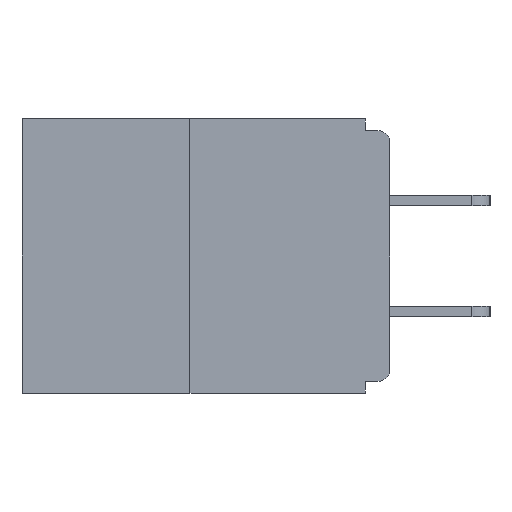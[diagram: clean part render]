
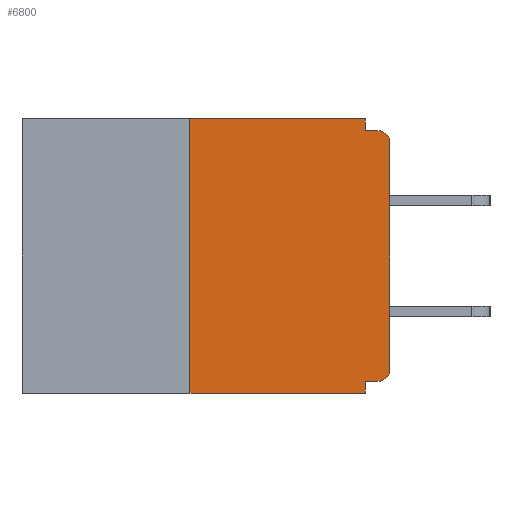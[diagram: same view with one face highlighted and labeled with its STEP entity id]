
A CAD part, left-side view. The second image highlights one B-rep face of the part: STEP entity #6800.
In plain terms, the highlighted planar face has unit normal (-1, 0, 0).
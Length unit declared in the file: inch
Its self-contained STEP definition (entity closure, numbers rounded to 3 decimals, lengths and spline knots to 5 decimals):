
#405 = DIRECTION ( 'NONE',  ( 0., -1., 0. ) ) ;
#660 = EDGE_CURVE ( 'NONE', #5271, #11070, #5580, .T. ) ;
#1061 = ORIENTED_EDGE ( 'NONE', *, *, #18727, .T. ) ;
#1547 = CARTESIAN_POINT ( 'NONE',  ( 0., 0.031, -0.015 ) ) ;
#1604 = DIRECTION ( 'NONE',  ( 0., 0., -1. ) ) ;
#2014 = AXIS2_PLACEMENT_3D ( 'NONE', #5248, #11078, #9657 ) ;
#2250 = VECTOR ( 'NONE', #5991, 39.37008 ) ;
#2292 = ORIENTED_EDGE ( 'NONE', *, *, #6930, .T. ) ;
#2561 = PLANE ( 'NONE',  #9073 ) ;
#3020 = CARTESIAN_POINT ( 'NONE',  ( 0., 0.015, -0.313 ) ) ;
#3096 = EDGE_CURVE ( 'NONE', #10043, #10060, #14631, .T. ) ;
#3568 = LINE ( 'NONE', #4851, #5735 ) ;
#3591 = ORIENTED_EDGE ( 'NONE', *, *, #660, .T. ) ;
#3662 = VECTOR ( 'NONE', #7138, 39.37008 ) ;
#3813 = EDGE_CURVE ( 'NONE', #8362, #7101, #16430, .T. ) ;
#4395 = EDGE_CURVE ( 'NONE', #10060, #13598, #16961, .T. ) ;
#4552 = CARTESIAN_POINT ( 'NONE',  ( 0., 0.46, 0. ) ) ;
#4698 = ORIENTED_EDGE ( 'NONE', *, *, #3096, .F. ) ;
#4843 = LINE ( 'NONE', #4552, #2250 ) ;
#4851 = CARTESIAN_POINT ( 'NONE',  ( 0., 0.031, 0. ) ) ;
#5020 = CARTESIAN_POINT ( 'NONE',  ( 0., 0.25, 0. ) ) ;
#5248 = CARTESIAN_POINT ( 'NONE',  ( 0., 0.015, -0.03 ) ) ;
#5271 = VERTEX_POINT ( 'NONE', #17336 ) ;
#5580 = LINE ( 'NONE', #8769, #11493 ) ;
#5625 = DIRECTION ( 'NONE',  ( 1., 0., 0. ) ) ;
#5735 = VECTOR ( 'NONE', #15248, 39.37008 ) ;
#5991 = DIRECTION ( 'NONE',  ( 0., -1., 0. ) ) ;
#6041 = ORIENTED_EDGE ( 'NONE', *, *, #9148, .T. ) ;
#6800 = ADVANCED_FACE ( 'NONE', ( #18742 ), #2561, .F. ) ;
#6930 = EDGE_CURVE ( 'NONE', #11070, #7101, #14533, .T. ) ;
#6936 = CIRCLE ( 'NONE', #8808, 0.015 ) ;
#6983 = CARTESIAN_POINT ( 'NONE',  ( 0., 0.031, -0.328 ) ) ;
#7101 = VERTEX_POINT ( 'NONE', #8712 ) ;
#7138 = DIRECTION ( 'NONE',  ( 0., -1., 0. ) ) ;
#7335 = CARTESIAN_POINT ( 'NONE',  ( 0., 0.46, -0.343 ) ) ;
#7573 = CARTESIAN_POINT ( 'NONE',  ( 0., 0., -0.328 ) ) ;
#7575 = ORIENTED_EDGE ( 'NONE', *, *, #3813, .F. ) ;
#8362 = VERTEX_POINT ( 'NONE', #1547 ) ;
#8712 = CARTESIAN_POINT ( 'NONE',  ( 0., 0.015, -0.015 ) ) ;
#8769 = CARTESIAN_POINT ( 'NONE',  ( 0., 0., 0. ) ) ;
#8808 = AXIS2_PLACEMENT_3D ( 'NONE', #3020, #14703, #1604 ) ;
#8930 = CARTESIAN_POINT ( 'NONE',  ( 0., 0.25, -0.343 ) ) ;
#9073 = AXIS2_PLACEMENT_3D ( 'NONE', #9745, #5625, #14139 ) ;
#9148 = EDGE_CURVE ( 'NONE', #10219, #13598, #18723, .T. ) ;
#9657 = DIRECTION ( 'NONE',  ( 0., 0., -1. ) ) ;
#9745 = CARTESIAN_POINT ( 'NONE',  ( 0., 0.46, 0. ) ) ;
#9764 = CARTESIAN_POINT ( 'NONE',  ( 0., 0.015, -0.328 ) ) ;
#10043 = VERTEX_POINT ( 'NONE', #9764 ) ;
#10060 = VERTEX_POINT ( 'NONE', #6983 ) ;
#10219 = VERTEX_POINT ( 'NONE', #8930 ) ;
#10251 = VECTOR ( 'NONE', #11140, 39.37008 ) ;
#10280 = DIRECTION ( 'NONE',  ( 0., 0., 1. ) ) ;
#10367 = CARTESIAN_POINT ( 'NONE',  ( 0., 0., -0.03 ) ) ;
#10816 = VECTOR ( 'NONE', #16054, 39.37008 ) ;
#11070 = VERTEX_POINT ( 'NONE', #10367 ) ;
#11078 = DIRECTION ( 'NONE',  ( -1., 0., 0. ) ) ;
#11140 = DIRECTION ( 'NONE',  ( 0., 0., -1. ) ) ;
#11180 = VERTEX_POINT ( 'NONE', #13701 ) ;
#11493 = VECTOR ( 'NONE', #10280, 39.37008 ) ;
#12693 = VECTOR ( 'NONE', #405, 39.37008 ) ;
#12928 = VECTOR ( 'NONE', #18211, 39.37008 ) ;
#13598 = VERTEX_POINT ( 'NONE', #17643 ) ;
#13669 = CARTESIAN_POINT ( 'NONE',  ( 0., 0., -0.015 ) ) ;
#13701 = CARTESIAN_POINT ( 'NONE',  ( 0., 0.031, 0. ) ) ;
#13817 = LINE ( 'NONE', #5020, #12928 ) ;
#13837 = ORIENTED_EDGE ( 'NONE', *, *, #4395, .F. ) ;
#13941 = ORIENTED_EDGE ( 'NONE', *, *, #18836, .F. ) ;
#14139 = DIRECTION ( 'NONE',  ( 0., 0., -1. ) ) ;
#14533 = CIRCLE ( 'NONE', #2014, 0.015 ) ;
#14590 = ORIENTED_EDGE ( 'NONE', *, *, #14895, .F. ) ;
#14607 = CARTESIAN_POINT ( 'NONE',  ( 0., 0.25, 0. ) ) ;
#14631 = LINE ( 'NONE', #7573, #10816 ) ;
#14703 = DIRECTION ( 'NONE',  ( -1., 0., 0. ) ) ;
#14787 = EDGE_CURVE ( 'NONE', #18623, #11180, #4843, .T. ) ;
#14895 = EDGE_CURVE ( 'NONE', #10219, #18623, #13817, .T. ) ;
#15248 = DIRECTION ( 'NONE',  ( 0., 0., -1. ) ) ;
#16054 = DIRECTION ( 'NONE',  ( 0., 1., 0. ) ) ;
#16430 = LINE ( 'NONE', #13669, #12693 ) ;
#16961 = LINE ( 'NONE', #17048, #10251 ) ;
#17048 = CARTESIAN_POINT ( 'NONE',  ( 0., 0.031, -0.343 ) ) ;
#17336 = CARTESIAN_POINT ( 'NONE',  ( 0., 0., -0.313 ) ) ;
#17578 = ORIENTED_EDGE ( 'NONE', *, *, #14787, .F. ) ;
#17643 = CARTESIAN_POINT ( 'NONE',  ( 0., 0.031, -0.343 ) ) ;
#18211 = DIRECTION ( 'NONE',  ( 0., 0., 1. ) ) ;
#18320 = EDGE_LOOP ( 'NONE', ( #17578, #14590, #6041, #13837, #4698, #1061, #3591, #2292, #7575, #13941 ) ) ;
#18623 = VERTEX_POINT ( 'NONE', #14607 ) ;
#18723 = LINE ( 'NONE', #7335, #3662 ) ;
#18727 = EDGE_CURVE ( 'NONE', #10043, #5271, #6936, .T. ) ;
#18742 = FACE_OUTER_BOUND ( 'NONE', #18320, .T. ) ;
#18836 = EDGE_CURVE ( 'NONE', #11180, #8362, #3568, .T. ) ;
